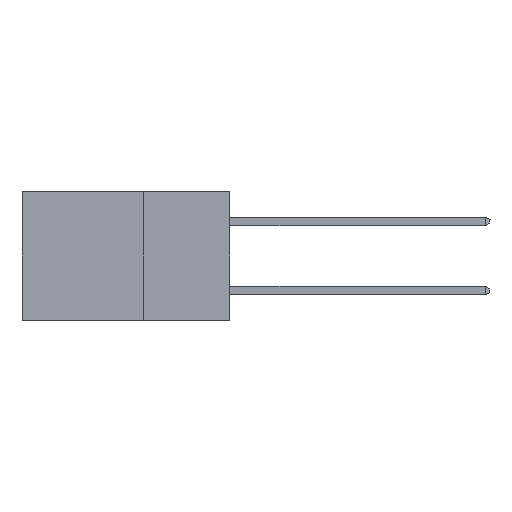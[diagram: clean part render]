
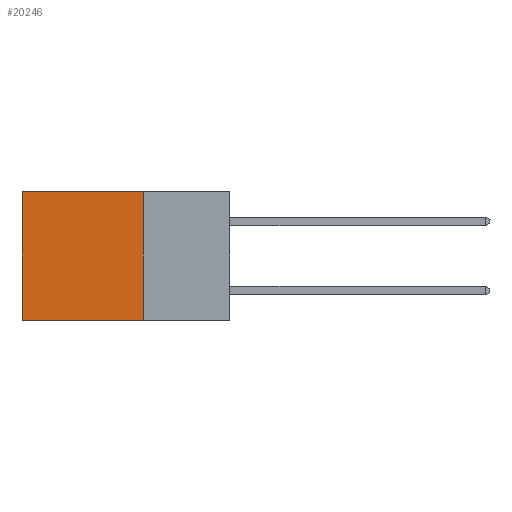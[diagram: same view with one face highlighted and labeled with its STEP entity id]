
A CAD part, left-side view. The second image highlights one B-rep face of the part: STEP entity #20246.
In plain terms, the highlighted planar face has unit normal (-1, 0, 0).
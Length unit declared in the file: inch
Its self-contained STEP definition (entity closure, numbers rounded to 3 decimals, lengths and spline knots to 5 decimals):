
#936 = ORIENTED_EDGE ( 'NONE', *, *, #23378, .T. ) ;
#3218 = CARTESIAN_POINT ( 'NONE',  ( 0.298, 0.6, 0. ) ) ;
#4047 = LINE ( 'NONE', #23752, #15613 ) ;
#4132 = DIRECTION ( 'NONE',  ( 0., 1., 0. ) ) ;
#4392 = CARTESIAN_POINT ( 'NONE',  ( 0.298, 0.25, 0. ) ) ;
#5319 = CARTESIAN_POINT ( 'NONE',  ( 0.298, 0.6, -0.37 ) ) ;
#8351 = VERTEX_POINT ( 'NONE', #15908 ) ;
#9569 = VECTOR ( 'NONE', #14887, 39.37008 ) ;
#10053 = ORIENTED_EDGE ( 'NONE', *, *, #12188, .F. ) ;
#10771 = ORIENTED_EDGE ( 'NONE', *, *, #27925, .F. ) ;
#10828 = VECTOR ( 'NONE', #30230, 39.37008 ) ;
#12188 = EDGE_CURVE ( 'NONE', #28223, #24765, #16905, .T. ) ;
#12315 = DIRECTION ( 'NONE',  ( 1., 0., 0. ) ) ;
#14199 = FACE_OUTER_BOUND ( 'NONE', #22491, .T. ) ;
#14827 = EDGE_CURVE ( 'NONE', #28223, #8351, #4047, .T. ) ;
#14887 = DIRECTION ( 'NONE',  ( 0., 0., -1. ) ) ;
#15613 = VECTOR ( 'NONE', #4132, 39.37008 ) ;
#15908 = CARTESIAN_POINT ( 'NONE',  ( 0.298, 0.6, 0. ) ) ;
#16905 = LINE ( 'NONE', #19846, #9569 ) ;
#18834 = VECTOR ( 'NONE', #22961, 39.37008 ) ;
#19654 = PLANE ( 'NONE',  #28740 ) ;
#19846 = CARTESIAN_POINT ( 'NONE',  ( 0.298, 0.25, 0. ) ) ;
#20246 = ADVANCED_FACE ( 'NONE', ( #14199 ), #19654, .F. ) ;
#22491 = EDGE_LOOP ( 'NONE', ( #936, #10771, #10053, #29950 ) ) ;
#22961 = DIRECTION ( 'NONE',  ( 0., 0., -1. ) ) ;
#23098 = CARTESIAN_POINT ( 'NONE',  ( 0.298, 0.25, -0.37 ) ) ;
#23378 = EDGE_CURVE ( 'NONE', #8351, #24633, #26083, .T. ) ;
#23752 = CARTESIAN_POINT ( 'NONE',  ( 0.298, 0.25, 0. ) ) ;
#23931 = LINE ( 'NONE', #27784, #10828 ) ;
#24633 = VERTEX_POINT ( 'NONE', #5319 ) ;
#24765 = VERTEX_POINT ( 'NONE', #23098 ) ;
#26083 = LINE ( 'NONE', #3218, #18834 ) ;
#26977 = CARTESIAN_POINT ( 'NONE',  ( 0.298, 0.25, 0. ) ) ;
#27784 = CARTESIAN_POINT ( 'NONE',  ( 0.298, 0.25, -0.37 ) ) ;
#27925 = EDGE_CURVE ( 'NONE', #24765, #24633, #23931, .T. ) ;
#28223 = VERTEX_POINT ( 'NONE', #4392 ) ;
#28740 = AXIS2_PLACEMENT_3D ( 'NONE', #26977, #12315, #29431 ) ;
#29431 = DIRECTION ( 'NONE',  ( 0., 0., -1. ) ) ;
#29950 = ORIENTED_EDGE ( 'NONE', *, *, #14827, .T. ) ;
#30230 = DIRECTION ( 'NONE',  ( 0., 1., 0. ) ) ;
